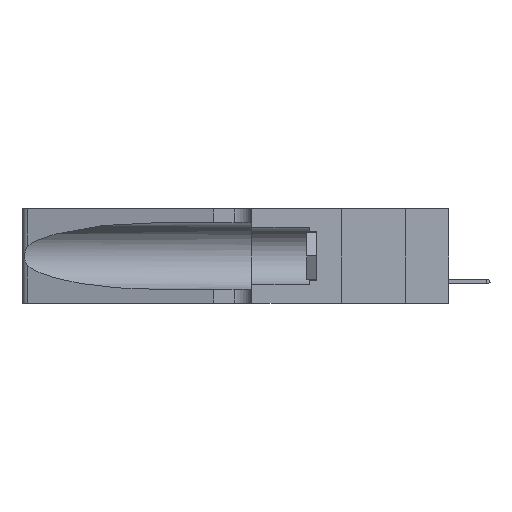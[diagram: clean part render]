
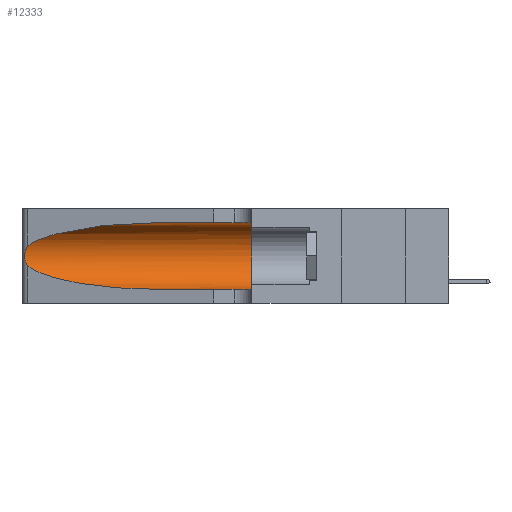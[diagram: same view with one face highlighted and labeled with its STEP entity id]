
A CAD part, left-side view. The second image highlights one B-rep face of the part: STEP entity #12333.
In plain terms, the highlighted cylindrical face has radius 3.308 mm (diameter 6.617 mm), a partial arc.
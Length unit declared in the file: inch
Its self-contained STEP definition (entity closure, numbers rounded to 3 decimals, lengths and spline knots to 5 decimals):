
#29 = ORIENTED_EDGE ( 'NONE', *, *, #379, .F. ) ;
#31 = CARTESIAN_POINT ( 'NONE',  ( 0.18966, 0.96281, 0.31525 ) ) ;
#222 = CARTESIAN_POINT ( 'NONE',  ( 0.1305, 0.35, 0.185 ) ) ;
#379 = EDGE_CURVE ( 'NONE', #30033, #27208, #23179, .T. ) ;
#635 = CARTESIAN_POINT ( 'NONE',  ( 0.1305, 1.61858, 0.185 ) ) ;
#915 = CARTESIAN_POINT ( 'NONE',  ( 0.1305, 0.72297, 0.05475 ) ) ;
#1051 = CARTESIAN_POINT ( 'NONE',  ( 0.26075, 1.23896, 0.178 ) ) ;
#2141 = LINE ( 'NONE', #12303, #6409 ) ;
#2171 = ORIENTED_EDGE ( 'NONE', *, *, #11078, .T. ) ;
#2239 = VECTOR ( 'NONE', #17689, 39.37008 ) ;
#2386 = DIRECTION ( 'NONE',  ( 0., 1., 0. ) ) ;
#3554 = CARTESIAN_POINT ( 'NONE',  ( 0.25487, 1.22718, 0.14631 ) ) ;
#4566 = EDGE_CURVE ( 'NONE', #27208, #11447, #6152, .T. ) ;
#6124 = FACE_OUTER_BOUND ( 'NONE', #17160, .T. ) ;
#6152 = CIRCLE ( 'NONE', #37887, 0.13025 ) ;
#6409 = VECTOR ( 'NONE', #15513, 39.37008 ) ;
#7424 = CARTESIAN_POINT ( 'NONE',  ( 0.1305, 0.72297, 0.31525 ) ) ;
#8304 = CARTESIAN_POINT ( 'NONE',  ( 0.1305, 0.35, 0.05475 ) ) ;
#8960 =( BOUNDED_CURVE ( )  B_SPLINE_CURVE ( 3, ( #33866, #31, #15369, #18656 ),
 .UNSPECIFIED., .F., .F. ) 
 B_SPLINE_CURVE_WITH_KNOTS ( ( 4, 4 ),
 ( 1.5708, 2.84003 ),
 .UNSPECIFIED. ) 
 CURVE ( )  GEOMETRIC_REPRESENTATION_ITEM ( )  RATIONAL_B_SPLINE_CURVE ( ( 1., 0.87, 0.87, 1. ) ) 
 REPRESENTATION_ITEM ( '' )  );
#9967 = CARTESIAN_POINT ( 'NONE',  ( 0.25487, 1.22718, 0.22369 ) ) ;
#10356 = CARTESIAN_POINT ( 'NONE',  ( 0.26075, 1.23896, 0.19203 ) ) ;
#11078 = EDGE_CURVE ( 'NONE', #20238, #24956, #18062, .T. ) ;
#11447 = VERTEX_POINT ( 'NONE', #8304 ) ;
#12303 = CARTESIAN_POINT ( 'NONE',  ( 0.1305, 1.61858, 0.05475 ) ) ;
#12333 = ADVANCED_FACE ( 'NONE', ( #6124 ), #22302, .F. ) ;
#12750 = DIRECTION ( 'NONE',  ( 0., 0., -1. ) ) ;
#13032 = CARTESIAN_POINT ( 'NONE',  ( 0.25854, 1.2359, 0.20912 ) ) ;
#13397 = EDGE_CURVE ( 'NONE', #30033, #26052, #8960, .T. ) ;
#14199 = CARTESIAN_POINT ( 'NONE',  ( 0.1305, 0.35, 0.31525 ) ) ;
#15369 = CARTESIAN_POINT ( 'NONE',  ( 0.2373, 1.15595, 0.28018 ) ) ;
#15398 = ORIENTED_EDGE ( 'NONE', *, *, #4566, .F. ) ;
#15513 = DIRECTION ( 'NONE',  ( 0., -1., 0. ) ) ;
#15966 = DIRECTION ( 'NONE',  ( 0., -1., 0. ) ) ;
#16373 = CARTESIAN_POINT ( 'NONE',  ( 0.25639, 1.23186, 0.15144 ) ) ;
#17160 = EDGE_LOOP ( 'NONE', ( #20077, #24038, #2171, #25846, #15398, #29 ) ) ;
#17689 = DIRECTION ( 'NONE',  ( 0., -1., 0. ) ) ;
#17937 = CARTESIAN_POINT ( 'NONE',  ( 0.1305, 1.61858, 0.31525 ) ) ;
#18062 =( BOUNDED_CURVE ( )  B_SPLINE_CURVE ( 3, ( #3554, #30993, #27502, #34037 ),
 .UNSPECIFIED., .F., .F. ) 
 B_SPLINE_CURVE_WITH_KNOTS ( ( 4, 4 ),
 ( 3.44316, 4.71239 ),
 .UNSPECIFIED. ) 
 CURVE ( )  GEOMETRIC_REPRESENTATION_ITEM ( )  RATIONAL_B_SPLINE_CURVE ( ( 1., 0.87, 0.87, 1. ) ) 
 REPRESENTATION_ITEM ( '' )  );
#18656 = CARTESIAN_POINT ( 'NONE',  ( 0.25487, 1.22718, 0.22369 ) ) ;
#19209 = AXIS2_PLACEMENT_3D ( 'NONE', #635, #15966, #12750 ) ;
#19292 = CARTESIAN_POINT ( 'NONE',  ( 0.25787, 1.23484, 0.2124 ) ) ;
#19411 = CARTESIAN_POINT ( 'NONE',  ( 0.25555, 1.22993, 0.14849 ) ) ;
#19547 = CARTESIAN_POINT ( 'NONE',  ( 0.25487, 1.22718, 0.14631 ) ) ;
#20077 = ORIENTED_EDGE ( 'NONE', *, *, #13397, .T. ) ;
#20238 = VERTEX_POINT ( 'NONE', #31042 ) ;
#22302 = CYLINDRICAL_SURFACE ( 'NONE', #19209, 0.13025 ) ;
#23153 = EDGE_CURVE ( 'NONE', #26052, #20238, #27978, .T. ) ;
#23179 = LINE ( 'NONE', #17937, #2239 ) ;
#23659 = DIRECTION ( 'NONE',  ( 0., 0., 1. ) ) ;
#24038 = ORIENTED_EDGE ( 'NONE', *, *, #23153, .T. ) ;
#24956 = VERTEX_POINT ( 'NONE', #915 ) ;
#25846 = ORIENTED_EDGE ( 'NONE', *, *, #27535, .T. ) ;
#26052 = VERTEX_POINT ( 'NONE', #26145 ) ;
#26145 = CARTESIAN_POINT ( 'NONE',  ( 0.25487, 1.22718, 0.22369 ) ) ;
#27208 = VERTEX_POINT ( 'NONE', #14199 ) ;
#27502 = CARTESIAN_POINT ( 'NONE',  ( 0.18966, 0.96281, 0.05475 ) ) ;
#27535 = EDGE_CURVE ( 'NONE', #24956, #11447, #2141, .T. ) ;
#27978 = B_SPLINE_CURVE_WITH_KNOTS ( 'NONE', 3,
 ( #9967, #34502, #28613, #19292, #13032, #34372, #10356, #1051, #34634, #37472, #31719, #16373, #19411, #19547 ),
 .UNSPECIFIED., .F., .F.,
 ( 4, 2, 2, 2, 2, 2, 4 ),
 ( 0., 0.00027, 0.00053, 0.00107, 0.0016, 0.00187, 0.00214 ),
 .UNSPECIFIED. ) ;
#28613 = CARTESIAN_POINT ( 'NONE',  ( 0.25639, 1.23184, 0.21858 ) ) ;
#30033 = VERTEX_POINT ( 'NONE', #7424 ) ;
#30993 = CARTESIAN_POINT ( 'NONE',  ( 0.2373, 1.15595, 0.08982 ) ) ;
#31042 = CARTESIAN_POINT ( 'NONE',  ( 0.25487, 1.22718, 0.14631 ) ) ;
#31719 = CARTESIAN_POINT ( 'NONE',  ( 0.25789, 1.23486, 0.15765 ) ) ;
#33866 = CARTESIAN_POINT ( 'NONE',  ( 0.1305, 0.72297, 0.31525 ) ) ;
#34037 = CARTESIAN_POINT ( 'NONE',  ( 0.1305, 0.72297, 0.05475 ) ) ;
#34372 = CARTESIAN_POINT ( 'NONE',  ( 0.26018, 1.23835, 0.19895 ) ) ;
#34502 = CARTESIAN_POINT ( 'NONE',  ( 0.25555, 1.22994, 0.2215 ) ) ;
#34634 = CARTESIAN_POINT ( 'NONE',  ( 0.26017, 1.23833, 0.17102 ) ) ;
#37472 = CARTESIAN_POINT ( 'NONE',  ( 0.25856, 1.23593, 0.16098 ) ) ;
#37887 = AXIS2_PLACEMENT_3D ( 'NONE', #222, #2386, #23659 ) ;
